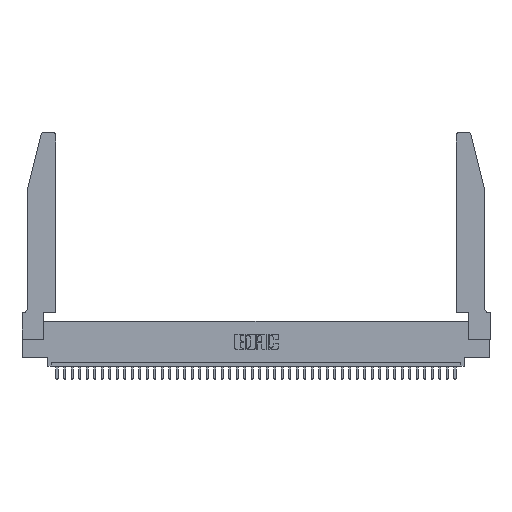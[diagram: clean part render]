
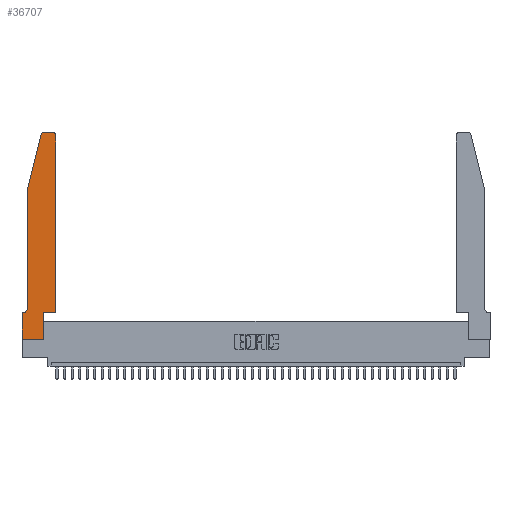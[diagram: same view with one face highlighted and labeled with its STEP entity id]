
A CAD part, top view. The second image highlights one B-rep face of the part: STEP entity #36707.
In plain terms, the highlighted planar face has unit normal (0, 0, 1).
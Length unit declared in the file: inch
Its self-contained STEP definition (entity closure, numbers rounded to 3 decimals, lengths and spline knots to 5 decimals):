
#494 = AXIS2_PLACEMENT_3D ( 'NONE', #10300, #3055, #36910 ) ;
#742 = CIRCLE ( 'NONE', #27280, 0.07 ) ;
#805 = VERTEX_POINT ( 'NONE', #38479 ) ;
#842 = VECTOR ( 'NONE', #23015, 39.37008 ) ;
#1051 = VECTOR ( 'NONE', #17948, 39.37008 ) ;
#1315 = DIRECTION ( 'NONE',  ( -0.239, -0.971, 0. ) ) ;
#2083 = DIRECTION ( 'NONE',  ( 0., -1., 0. ) ) ;
#2158 = ORIENTED_EDGE ( 'NONE', *, *, #11469, .T. ) ;
#2690 = LINE ( 'NONE', #43168, #21221 ) ;
#3055 = DIRECTION ( 'NONE',  ( 0., 0., 1. ) ) ;
#3093 = DIRECTION ( 'NONE',  ( -1., 0., 0. ) ) ;
#3601 = CARTESIAN_POINT ( 'NONE',  ( 0.0755, 0.42, 0.37 ) ) ;
#3710 = ORIENTED_EDGE ( 'NONE', *, *, #35924, .T. ) ;
#3811 = EDGE_CURVE ( 'NONE', #36998, #10564, #16784, .T. ) ;
#3881 = DIRECTION ( 'NONE',  ( 1., 0., 0. ) ) ;
#4151 = DIRECTION ( 'NONE',  ( 0., 0., 1. ) ) ;
#4328 = VERTEX_POINT ( 'NONE', #40211 ) ;
#4466 = EDGE_CURVE ( 'NONE', #19012, #13190, #742, .T. ) ;
#5345 = VECTOR ( 'NONE', #39637, 39.37008 ) ;
#5573 = VERTEX_POINT ( 'NONE', #36638 ) ;
#6264 = VECTOR ( 'NONE', #18875, 39.37008 ) ;
#6467 = CARTESIAN_POINT ( 'NONE',  ( 0.4505, 0.35, 0.37 ) ) ;
#8795 = CARTESIAN_POINT ( 'NONE',  ( 0.2865, 0.35, 0.37 ) ) ;
#8947 = CIRCLE ( 'NONE', #494, 0.03 ) ;
#9705 = DIRECTION ( 'NONE',  ( -1., 0., 0. ) ) ;
#10266 = CARTESIAN_POINT ( 'NONE',  ( 0.25487, 2.72718, 0.37 ) ) ;
#10300 = CARTESIAN_POINT ( 'NONE',  ( 0.4205, 2.72, 0.37 ) ) ;
#10564 = VERTEX_POINT ( 'NONE', #6467 ) ;
#11469 = EDGE_CURVE ( 'NONE', #12953, #32936, #28244, .T. ) ;
#12113 = AXIS2_PLACEMENT_3D ( 'NONE', #21213, #4151, #3881 ) ;
#12241 = ORIENTED_EDGE ( 'NONE', *, *, #43392, .T. ) ;
#12331 = EDGE_CURVE ( 'NONE', #805, #43445, #22318, .T. ) ;
#12712 = DIRECTION ( 'NONE',  ( 0., 0., 1. ) ) ;
#12766 = CARTESIAN_POINT ( 'NONE',  ( 0.0755, 2., 0.37 ) ) ;
#12953 = VERTEX_POINT ( 'NONE', #10266 ) ;
#13018 = VERTEX_POINT ( 'NONE', #27603 ) ;
#13108 = CARTESIAN_POINT ( 'NONE',  ( 0., 0., 0.37 ) ) ;
#13190 = VERTEX_POINT ( 'NONE', #31297 ) ;
#14512 = EDGE_CURVE ( 'NONE', #4328, #805, #29878, .T. ) ;
#15704 = EDGE_CURVE ( 'NONE', #10564, #13018, #23408, .T. ) ;
#16752 = VECTOR ( 'NONE', #41658, 39.37008 ) ;
#16784 = LINE ( 'NONE', #34873, #18371 ) ;
#17099 = ORIENTED_EDGE ( 'NONE', *, *, #3811, .T. ) ;
#17463 = EDGE_LOOP ( 'NONE', ( #37557, #42963, #2158, #12241, #31222, #3710, #42769, #30040, #43716, #17099, #43360, #34071 ) ) ;
#17948 = DIRECTION ( 'NONE',  ( 1., 0., 0. ) ) ;
#18098 = DIRECTION ( 'NONE',  ( 1., 0., 0. ) ) ;
#18371 = VECTOR ( 'NONE', #18098, 39.37008 ) ;
#18875 = DIRECTION ( 'NONE',  ( 0., 1., 0. ) ) ;
#19012 = VERTEX_POINT ( 'NONE', #3601 ) ;
#20387 = CARTESIAN_POINT ( 'NONE',  ( 0.2605, 2.75, 0.37 ) ) ;
#20513 = CARTESIAN_POINT ( 'NONE',  ( 0.4205, 2.75, 0.37 ) ) ;
#20917 = CARTESIAN_POINT ( 'NONE',  ( 0., 0., 0.37 ) ) ;
#21213 = CARTESIAN_POINT ( 'NONE',  ( 0., 0.35, 0.37 ) ) ;
#21221 = VECTOR ( 'NONE', #9705, 39.37008 ) ;
#22105 = LINE ( 'NONE', #36552, #842 ) ;
#22318 = LINE ( 'NONE', #20917, #1051 ) ;
#23015 = DIRECTION ( 'NONE',  ( 0., -1., 0. ) ) ;
#23075 = DIRECTION ( 'NONE',  ( 1., 0., 0. ) ) ;
#23119 = LINE ( 'NONE', #20387, #16752 ) ;
#23127 = EDGE_CURVE ( 'NONE', #43445, #36998, #31733, .T. ) ;
#23346 = FACE_OUTER_BOUND ( 'NONE', #17463, .T. ) ;
#23408 = LINE ( 'NONE', #35739, #5345 ) ;
#26110 = CARTESIAN_POINT ( 'NONE',  ( 0.2865, 0., 0.37 ) ) ;
#26830 = DIRECTION ( 'NONE',  ( 0., 0., -1. ) ) ;
#27280 = AXIS2_PLACEMENT_3D ( 'NONE', #43784, #26830, #3093 ) ;
#27603 = CARTESIAN_POINT ( 'NONE',  ( 0.4505, 2.72, 0.37 ) ) ;
#28244 = LINE ( 'NONE', #41486, #35154 ) ;
#28954 = EDGE_CURVE ( 'NONE', #13018, #36518, #8947, .T. ) ;
#29878 = LINE ( 'NONE', #13108, #34644 ) ;
#30040 = ORIENTED_EDGE ( 'NONE', *, *, #12331, .T. ) ;
#30713 = EDGE_CURVE ( 'NONE', #5573, #12953, #33805, .T. ) ;
#31222 = ORIENTED_EDGE ( 'NONE', *, *, #4466, .T. ) ;
#31297 = CARTESIAN_POINT ( 'NONE',  ( 0.0055, 0.35, 0.37 ) ) ;
#31733 = LINE ( 'NONE', #8795, #6264 ) ;
#32648 = EDGE_CURVE ( 'NONE', #36518, #5573, #23119, .T. ) ;
#32936 = VERTEX_POINT ( 'NONE', #12766 ) ;
#33805 = CIRCLE ( 'NONE', #34164, 0.03 ) ;
#34071 = ORIENTED_EDGE ( 'NONE', *, *, #28954, .T. ) ;
#34164 = AXIS2_PLACEMENT_3D ( 'NONE', #40506, #12712, #23075 ) ;
#34467 = PLANE ( 'NONE',  #12113 ) ;
#34644 = VECTOR ( 'NONE', #2083, 39.37008 ) ;
#34873 = CARTESIAN_POINT ( 'NONE',  ( 0.4505, 0.35, 0.37 ) ) ;
#35154 = VECTOR ( 'NONE', #1315, 39.37008 ) ;
#35632 = CARTESIAN_POINT ( 'NONE',  ( 0.2865, 0.35, 0.37 ) ) ;
#35739 = CARTESIAN_POINT ( 'NONE',  ( 0.4505, 0.35, 0.37 ) ) ;
#35924 = EDGE_CURVE ( 'NONE', #13190, #4328, #2690, .T. ) ;
#36518 = VERTEX_POINT ( 'NONE', #20513 ) ;
#36552 = CARTESIAN_POINT ( 'NONE',  ( 0.0755, 2., 0.37 ) ) ;
#36638 = CARTESIAN_POINT ( 'NONE',  ( 0.284, 2.75, 0.37 ) ) ;
#36707 = ADVANCED_FACE ( 'NONE', ( #23346 ), #34467, .T. ) ;
#36910 = DIRECTION ( 'NONE',  ( 1., 0., 0. ) ) ;
#36998 = VERTEX_POINT ( 'NONE', #35632 ) ;
#37557 = ORIENTED_EDGE ( 'NONE', *, *, #32648, .T. ) ;
#38479 = CARTESIAN_POINT ( 'NONE',  ( 0., 0., 0.37 ) ) ;
#39637 = DIRECTION ( 'NONE',  ( 0., 1., 0. ) ) ;
#40211 = CARTESIAN_POINT ( 'NONE',  ( 0., 0.35, 0.37 ) ) ;
#40506 = CARTESIAN_POINT ( 'NONE',  ( 0.284, 2.72, 0.37 ) ) ;
#41486 = CARTESIAN_POINT ( 'NONE',  ( 0.0755, 2., 0.37 ) ) ;
#41658 = DIRECTION ( 'NONE',  ( -1., 0., 0. ) ) ;
#42769 = ORIENTED_EDGE ( 'NONE', *, *, #14512, .T. ) ;
#42963 = ORIENTED_EDGE ( 'NONE', *, *, #30713, .T. ) ;
#43168 = CARTESIAN_POINT ( 'NONE',  ( 0.0755, 0.35, 0.37 ) ) ;
#43360 = ORIENTED_EDGE ( 'NONE', *, *, #15704, .T. ) ;
#43392 = EDGE_CURVE ( 'NONE', #32936, #19012, #22105, .T. ) ;
#43445 = VERTEX_POINT ( 'NONE', #26110 ) ;
#43716 = ORIENTED_EDGE ( 'NONE', *, *, #23127, .T. ) ;
#43784 = CARTESIAN_POINT ( 'NONE',  ( 0.0055, 0.42, 0.37 ) ) ;
